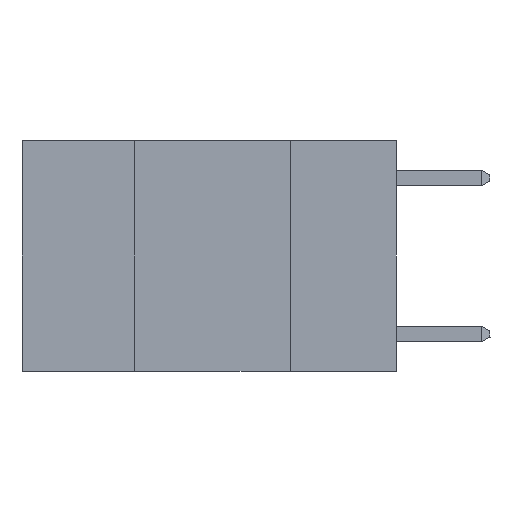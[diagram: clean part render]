
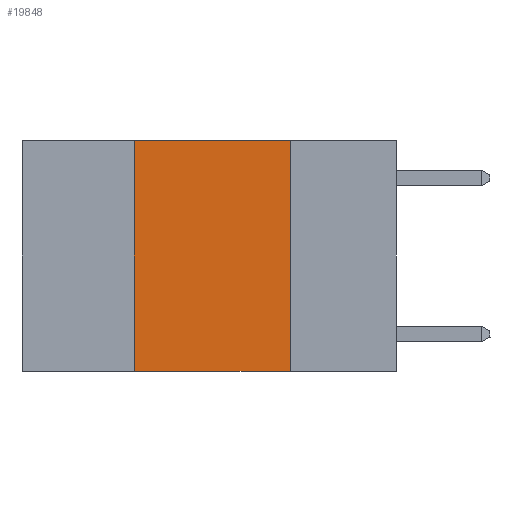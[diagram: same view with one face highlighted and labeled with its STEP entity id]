
A CAD part, left-side view. The second image highlights one B-rep face of the part: STEP entity #19848.
In plain terms, the highlighted planar face has unit normal (-1, 0, 0).
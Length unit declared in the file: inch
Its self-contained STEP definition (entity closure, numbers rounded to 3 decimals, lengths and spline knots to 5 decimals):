
#131 = ORIENTED_EDGE ( 'NONE', *, *, #5051, .F. ) ;
#152 = ORIENTED_EDGE ( 'NONE', *, *, #14628, .T. ) ;
#189 = VECTOR ( 'NONE', #8323, 39.37008 ) ;
#312 = EDGE_CURVE ( 'NONE', #21923, #22233, #431, .T. ) ;
#431 = LINE ( 'NONE', #12781, #189 ) ;
#718 = PLANE ( 'NONE',  #23240 ) ;
#1144 = EDGE_LOOP ( 'NONE', ( #24018, #24120, #131, #152 ) ) ;
#1163 = VECTOR ( 'NONE', #18714, 39.37008 ) ;
#1387 = LINE ( 'NONE', #16855, #1163 ) ;
#2084 = CARTESIAN_POINT ( 'NONE',  ( 0., 0.17, 0. ) ) ;
#2817 = DIRECTION ( 'NONE',  ( 0., -1., 0. ) ) ;
#4184 = EDGE_CURVE ( 'NONE', #22233, #4661, #7058, .T. ) ;
#4661 = VERTEX_POINT ( 'NONE', #17671 ) ;
#5051 = EDGE_CURVE ( 'NONE', #12694, #21923, #1387, .T. ) ;
#5578 = CARTESIAN_POINT ( 'NONE',  ( 0., 0.17, 0. ) ) ;
#7058 = LINE ( 'NONE', #2084, #7173 ) ;
#7173 = VECTOR ( 'NONE', #10663, 39.37008 ) ;
#8323 = DIRECTION ( 'NONE',  ( 0., -1., 0. ) ) ;
#8463 = DIRECTION ( 'NONE',  ( 0., 0., -1. ) ) ;
#10663 = DIRECTION ( 'NONE',  ( 0., 0., -1. ) ) ;
#12394 = CARTESIAN_POINT ( 'NONE',  ( 0., 0.6, -0.37 ) ) ;
#12694 = VERTEX_POINT ( 'NONE', #13009 ) ;
#12781 = CARTESIAN_POINT ( 'NONE',  ( 0., 0.6, 0. ) ) ;
#12972 = LINE ( 'NONE', #12394, #13143 ) ;
#13009 = CARTESIAN_POINT ( 'NONE',  ( 0., 0.42, -0.37 ) ) ;
#13143 = VECTOR ( 'NONE', #2817, 39.37008 ) ;
#14628 = EDGE_CURVE ( 'NONE', #12694, #4661, #12972, .T. ) ;
#14994 = FACE_OUTER_BOUND ( 'NONE', #1144, .T. ) ;
#16855 = CARTESIAN_POINT ( 'NONE',  ( 0., 0.42, 0. ) ) ;
#17671 = CARTESIAN_POINT ( 'NONE',  ( 0., 0.17, -0.37 ) ) ;
#18714 = DIRECTION ( 'NONE',  ( 0., 0., 1. ) ) ;
#19692 = CARTESIAN_POINT ( 'NONE',  ( 0., 0.42, 0. ) ) ;
#19813 = DIRECTION ( 'NONE',  ( 1., 0., 0. ) ) ;
#19848 = ADVANCED_FACE ( 'NONE', ( #14994 ), #718, .F. ) ;
#21923 = VERTEX_POINT ( 'NONE', #19692 ) ;
#22233 = VERTEX_POINT ( 'NONE', #5578 ) ;
#23240 = AXIS2_PLACEMENT_3D ( 'NONE', #23456, #19813, #8463 ) ;
#23456 = CARTESIAN_POINT ( 'NONE',  ( 0., 0.6, 0. ) ) ;
#24018 = ORIENTED_EDGE ( 'NONE', *, *, #4184, .F. ) ;
#24120 = ORIENTED_EDGE ( 'NONE', *, *, #312, .F. ) ;
